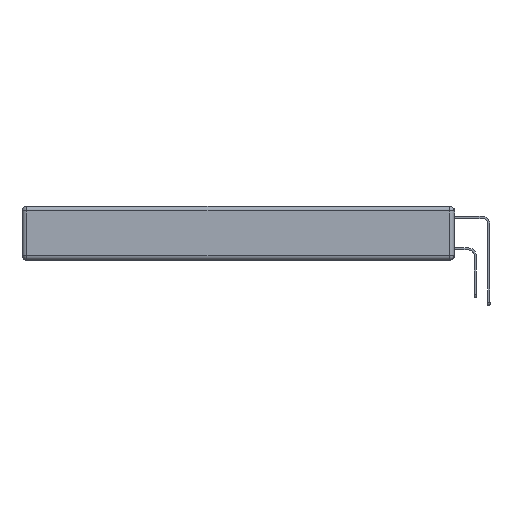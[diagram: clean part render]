
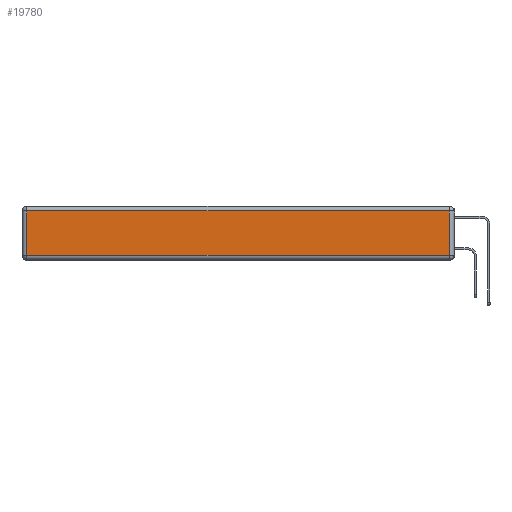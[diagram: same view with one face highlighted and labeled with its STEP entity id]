
A CAD part, left-side view. The second image highlights one B-rep face of the part: STEP entity #19780.
In plain terms, the highlighted planar face has unit normal (-1, 0, 0).
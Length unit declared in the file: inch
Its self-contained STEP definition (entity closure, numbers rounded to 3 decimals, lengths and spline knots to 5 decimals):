
#2 = ORIENTED_EDGE ( 'NONE', *, *, #22932, .T. ) ;
#32 = CARTESIAN_POINT ( 'NONE',  ( 0., 0., -0.343 ) ) ;
#365 = EDGE_CURVE ( 'NONE', #8947, #6713, #12006, .T. ) ;
#1097 = DIRECTION ( 'NONE',  ( 0., -1., 0. ) ) ;
#1977 = FACE_OUTER_BOUND ( 'NONE', #14075, .T. ) ;
#2955 = LINE ( 'NONE', #11997, #10832 ) ;
#4592 = DIRECTION ( 'NONE',  ( 0., 1., 0. ) ) ;
#4740 = CARTESIAN_POINT ( 'NONE',  ( 0., 2.72, -0.03 ) ) ;
#6713 = VERTEX_POINT ( 'NONE', #27943 ) ;
#7537 = DIRECTION ( 'NONE',  ( 0., 0., 1. ) ) ;
#8947 = VERTEX_POINT ( 'NONE', #13944 ) ;
#9995 = LINE ( 'NONE', #23926, #16900 ) ;
#10293 = DIRECTION ( 'NONE',  ( 0., 0., -1. ) ) ;
#10832 = VECTOR ( 'NONE', #4592, 39.37008 ) ;
#11341 = VECTOR ( 'NONE', #1097, 39.37008 ) ;
#11997 = CARTESIAN_POINT ( 'NONE',  ( 0., 2.75, -0.03 ) ) ;
#12006 = LINE ( 'NONE', #12596, #12339 ) ;
#12177 = ORIENTED_EDGE ( 'NONE', *, *, #20380, .T. ) ;
#12239 = CARTESIAN_POINT ( 'NONE',  ( 0., 0., -0.313 ) ) ;
#12339 = VECTOR ( 'NONE', #7537, 39.37008 ) ;
#12596 = CARTESIAN_POINT ( 'NONE',  ( 0., 0.03, -0.343 ) ) ;
#13160 = EDGE_CURVE ( 'NONE', #13895, #24246, #9995, .T. ) ;
#13895 = VERTEX_POINT ( 'NONE', #4740 ) ;
#13944 = CARTESIAN_POINT ( 'NONE',  ( 0., 0.03, -0.313 ) ) ;
#14075 = EDGE_LOOP ( 'NONE', ( #2, #28616, #12177, #15442 ) ) ;
#14209 = CARTESIAN_POINT ( 'NONE',  ( 0., 2.72, -0.313 ) ) ;
#15442 = ORIENTED_EDGE ( 'NONE', *, *, #13160, .T. ) ;
#15923 = DIRECTION ( 'NONE',  ( 0., 0., 1. ) ) ;
#16900 = VECTOR ( 'NONE', #10293, 39.37008 ) ;
#17142 = LINE ( 'NONE', #12239, #11341 ) ;
#19780 = ADVANCED_FACE ( 'NONE', ( #1977 ), #20384, .T. ) ;
#20380 = EDGE_CURVE ( 'NONE', #6713, #13895, #2955, .T. ) ;
#20384 = PLANE ( 'NONE',  #21199 ) ;
#21199 = AXIS2_PLACEMENT_3D ( 'NONE', #32, #28980, #15923 ) ;
#22932 = EDGE_CURVE ( 'NONE', #24246, #8947, #17142, .T. ) ;
#23926 = CARTESIAN_POINT ( 'NONE',  ( 0., 2.72, -0.343 ) ) ;
#24246 = VERTEX_POINT ( 'NONE', #14209 ) ;
#27943 = CARTESIAN_POINT ( 'NONE',  ( 0., 0.03, -0.03 ) ) ;
#28616 = ORIENTED_EDGE ( 'NONE', *, *, #365, .T. ) ;
#28980 = DIRECTION ( 'NONE',  ( -1., 0., 0. ) ) ;
